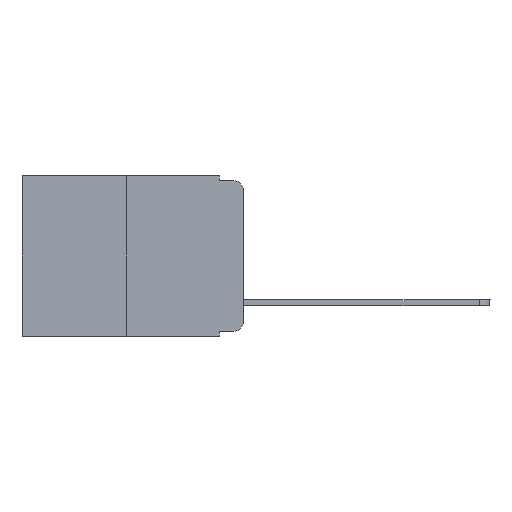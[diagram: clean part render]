
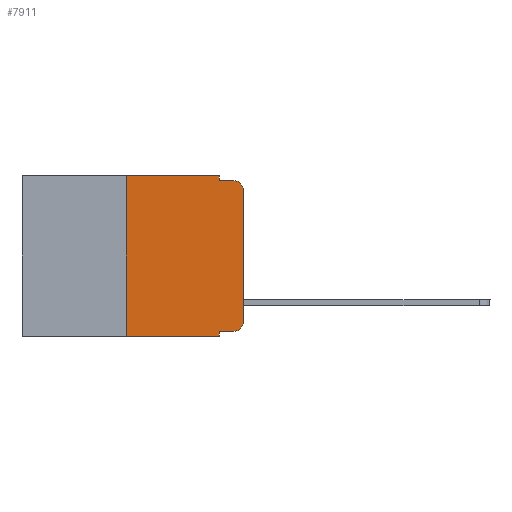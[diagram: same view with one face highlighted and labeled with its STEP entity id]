
A CAD part, left-side view. The second image highlights one B-rep face of the part: STEP entity #7911.
In plain terms, the highlighted planar face has unit normal (-1, 0, 0).
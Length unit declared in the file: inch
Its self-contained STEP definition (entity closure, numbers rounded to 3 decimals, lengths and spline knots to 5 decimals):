
#186 = DIRECTION ( 'NONE',  ( 0., 0., -1. ) ) ;
#534 = DIRECTION ( 'NONE',  ( 0., 0., 1. ) ) ;
#574 = VERTEX_POINT ( 'NONE', #3834 ) ;
#844 = CARTESIAN_POINT ( 'NONE',  ( 0., 0., 0. ) ) ;
#866 = DIRECTION ( 'NONE',  ( 0., -1., 0. ) ) ;
#1051 = EDGE_CURVE ( 'NONE', #574, #13191, #14861, .T. ) ;
#1134 = CIRCLE ( 'NONE', #5721, 0.02 ) ;
#1311 = CARTESIAN_POINT ( 'NONE',  ( 0., 0.051, 0. ) ) ;
#1493 = LINE ( 'NONE', #10171, #7336 ) ;
#1615 = LINE ( 'NONE', #5653, #3619 ) ;
#2040 = CARTESIAN_POINT ( 'NONE',  ( 0., 0.02, -0.03 ) ) ;
#2135 = DIRECTION ( 'NONE',  ( 0., 0., -1. ) ) ;
#2447 = DIRECTION ( 'NONE',  ( 0., 0., -1. ) ) ;
#2520 = EDGE_CURVE ( 'NONE', #8426, #10249, #1493, .T. ) ;
#2788 = CARTESIAN_POINT ( 'NONE',  ( 0., 0.051, -0.333 ) ) ;
#2991 = VECTOR ( 'NONE', #3394, 39.37008 ) ;
#3358 = CARTESIAN_POINT ( 'NONE',  ( 0., 0.02, -0.01 ) ) ;
#3394 = DIRECTION ( 'NONE',  ( 0., 0., -1. ) ) ;
#3479 = CARTESIAN_POINT ( 'NONE',  ( 0., 0.02, -0.313 ) ) ;
#3619 = VECTOR ( 'NONE', #12514, 39.37008 ) ;
#3715 = DIRECTION ( 'NONE',  ( 1., 0., 0. ) ) ;
#3722 = VECTOR ( 'NONE', #8713, 39.37008 ) ;
#3834 = CARTESIAN_POINT ( 'NONE',  ( 0., 0.25, -0.343 ) ) ;
#4391 = EDGE_CURVE ( 'NONE', #11071, #6672, #10581, .T. ) ;
#4643 = CARTESIAN_POINT ( 'NONE',  ( 0., 0.051, 0. ) ) ;
#4767 = ORIENTED_EDGE ( 'NONE', *, *, #7193, .F. ) ;
#5015 = ORIENTED_EDGE ( 'NONE', *, *, #7704, .T. ) ;
#5028 = EDGE_CURVE ( 'NONE', #574, #13764, #5061, .T. ) ;
#5061 = LINE ( 'NONE', #14822, #10736 ) ;
#5484 = DIRECTION ( 'NONE',  ( 0., -1., 0. ) ) ;
#5549 = CIRCLE ( 'NONE', #14876, 0.02 ) ;
#5653 = CARTESIAN_POINT ( 'NONE',  ( 0., 0.051, 0. ) ) ;
#5721 = AXIS2_PLACEMENT_3D ( 'NONE', #3479, #10428, #2447 ) ;
#5778 = ORIENTED_EDGE ( 'NONE', *, *, #2520, .F. ) ;
#6568 = VERTEX_POINT ( 'NONE', #1311 ) ;
#6672 = VERTEX_POINT ( 'NONE', #10859 ) ;
#6794 = ORIENTED_EDGE ( 'NONE', *, *, #12498, .T. ) ;
#6819 = LINE ( 'NONE', #4643, #2991 ) ;
#7193 = EDGE_CURVE ( 'NONE', #6568, #8426, #6819, .T. ) ;
#7195 = PLANE ( 'NONE',  #13281 ) ;
#7245 = LINE ( 'NONE', #844, #13102 ) ;
#7336 = VECTOR ( 'NONE', #866, 39.37008 ) ;
#7704 = EDGE_CURVE ( 'NONE', #6672, #12396, #1134, .T. ) ;
#7715 = CARTESIAN_POINT ( 'NONE',  ( 0., 0.25, 0. ) ) ;
#7911 = ADVANCED_FACE ( 'NONE', ( #11360 ), #7195, .F. ) ;
#7943 = CARTESIAN_POINT ( 'NONE',  ( 0., 0.051, -0.333 ) ) ;
#8007 = VERTEX_POINT ( 'NONE', #8669 ) ;
#8426 = VERTEX_POINT ( 'NONE', #11573 ) ;
#8461 = CARTESIAN_POINT ( 'NONE',  ( 0., 0.473, 0. ) ) ;
#8669 = CARTESIAN_POINT ( 'NONE',  ( 0., 0., -0.03 ) ) ;
#8713 = DIRECTION ( 'NONE',  ( 0., -1., 0. ) ) ;
#8786 = ORIENTED_EDGE ( 'NONE', *, *, #10619, .T. ) ;
#9946 = ORIENTED_EDGE ( 'NONE', *, *, #4391, .T. ) ;
#10171 = CARTESIAN_POINT ( 'NONE',  ( 0., 0.051, -0.01 ) ) ;
#10249 = VERTEX_POINT ( 'NONE', #3358 ) ;
#10358 = DIRECTION ( 'NONE',  ( 0., 0., 1. ) ) ;
#10428 = DIRECTION ( 'NONE',  ( -1., 0., 0. ) ) ;
#10484 = VECTOR ( 'NONE', #10358, 39.37008 ) ;
#10581 = LINE ( 'NONE', #7943, #15142 ) ;
#10619 = EDGE_CURVE ( 'NONE', #12396, #8007, #7245, .T. ) ;
#10736 = VECTOR ( 'NONE', #13611, 39.37008 ) ;
#10859 = CARTESIAN_POINT ( 'NONE',  ( 0., 0.02, -0.333 ) ) ;
#11071 = VERTEX_POINT ( 'NONE', #2788 ) ;
#11360 = FACE_OUTER_BOUND ( 'NONE', #15140, .T. ) ;
#11573 = CARTESIAN_POINT ( 'NONE',  ( 0., 0.051, -0.01 ) ) ;
#12345 = CARTESIAN_POINT ( 'NONE',  ( 0., 0.473, 0. ) ) ;
#12396 = VERTEX_POINT ( 'NONE', #13373 ) ;
#12414 = EDGE_CURVE ( 'NONE', #13191, #6568, #15053, .T. ) ;
#12498 = EDGE_CURVE ( 'NONE', #8007, #10249, #5549, .T. ) ;
#12514 = DIRECTION ( 'NONE',  ( 0., 0., -1. ) ) ;
#13102 = VECTOR ( 'NONE', #534, 39.37008 ) ;
#13191 = VERTEX_POINT ( 'NONE', #7715 ) ;
#13281 = AXIS2_PLACEMENT_3D ( 'NONE', #8461, #3715, #186 ) ;
#13373 = CARTESIAN_POINT ( 'NONE',  ( 0., 0., -0.313 ) ) ;
#13611 = DIRECTION ( 'NONE',  ( 0., -1., 0. ) ) ;
#13699 = CARTESIAN_POINT ( 'NONE',  ( 0., 0.051, -0.343 ) ) ;
#13764 = VERTEX_POINT ( 'NONE', #13699 ) ;
#13768 = ORIENTED_EDGE ( 'NONE', *, *, #1051, .F. ) ;
#13779 = EDGE_CURVE ( 'NONE', #11071, #13764, #1615, .T. ) ;
#13965 = ORIENTED_EDGE ( 'NONE', *, *, #12414, .F. ) ;
#14042 = ORIENTED_EDGE ( 'NONE', *, *, #5028, .T. ) ;
#14773 = ORIENTED_EDGE ( 'NONE', *, *, #13779, .F. ) ;
#14785 = DIRECTION ( 'NONE',  ( -1., 0., 0. ) ) ;
#14822 = CARTESIAN_POINT ( 'NONE',  ( 0., 0.473, -0.343 ) ) ;
#14861 = LINE ( 'NONE', #15093, #10484 ) ;
#14876 = AXIS2_PLACEMENT_3D ( 'NONE', #2040, #14785, #2135 ) ;
#15053 = LINE ( 'NONE', #12345, #3722 ) ;
#15093 = CARTESIAN_POINT ( 'NONE',  ( 0., 0.25, 0. ) ) ;
#15140 = EDGE_LOOP ( 'NONE', ( #8786, #6794, #5778, #4767, #13965, #13768, #14042, #14773, #9946, #5015 ) ) ;
#15142 = VECTOR ( 'NONE', #5484, 39.37008 ) ;
